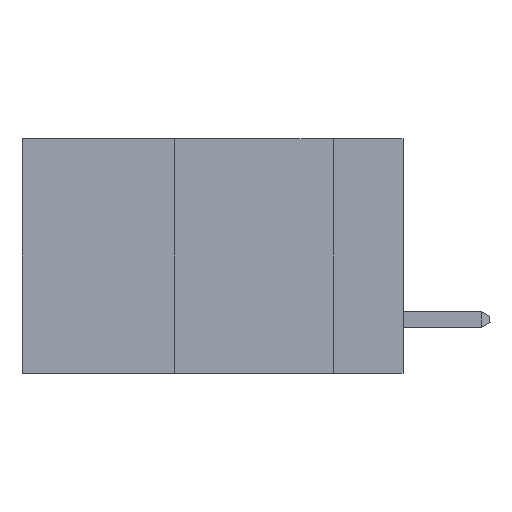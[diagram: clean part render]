
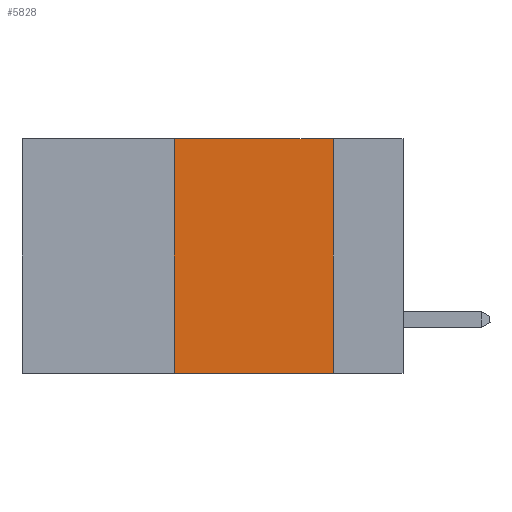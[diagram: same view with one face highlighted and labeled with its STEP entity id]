
A CAD part, left-side view. The second image highlights one B-rep face of the part: STEP entity #5828.
In plain terms, the highlighted planar face has unit normal (-1, 0, 0).
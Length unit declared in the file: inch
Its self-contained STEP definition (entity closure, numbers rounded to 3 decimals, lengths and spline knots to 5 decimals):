
#2307 = CARTESIAN_POINT ( 'NONE',  ( 0., 0.11, 0. ) ) ;
#2425 = CARTESIAN_POINT ( 'NONE',  ( 0., 0.36, 0. ) ) ;
#3149 = CARTESIAN_POINT ( 'NONE',  ( 0., 0.36, -0.37 ) ) ;
#4211 = VERTEX_POINT ( 'NONE', #2425 ) ;
#5221 = VERTEX_POINT ( 'NONE', #33621 ) ;
#5508 = CARTESIAN_POINT ( 'NONE',  ( 0., 0.6, 0. ) ) ;
#5828 = ADVANCED_FACE ( 'NONE', ( #44505 ), #46848, .F. ) ;
#6279 = CARTESIAN_POINT ( 'NONE',  ( 0., 0.11, -0.37 ) ) ;
#8503 = DIRECTION ( 'NONE',  ( 1., 0., 0. ) ) ;
#9434 = ORIENTED_EDGE ( 'NONE', *, *, #49886, .F. ) ;
#10566 = EDGE_CURVE ( 'NONE', #5221, #21000, #13052, .T. ) ;
#12055 = DIRECTION ( 'NONE',  ( 0., -1., 0. ) ) ;
#12700 = VECTOR ( 'NONE', #33296, 39.37008 ) ;
#13052 = LINE ( 'NONE', #2307, #20924 ) ;
#13953 = EDGE_LOOP ( 'NONE', ( #40912, #9434, #32445, #31749 ) ) ;
#14156 = DIRECTION ( 'NONE',  ( 0., 0., -1. ) ) ;
#17093 = EDGE_CURVE ( 'NONE', #43874, #21000, #49268, .T. ) ;
#20924 = VECTOR ( 'NONE', #14156, 39.37008 ) ;
#21000 = VERTEX_POINT ( 'NONE', #6279 ) ;
#21794 = CARTESIAN_POINT ( 'NONE',  ( 0., 0.36, 0. ) ) ;
#24425 = EDGE_CURVE ( 'NONE', #43874, #4211, #36939, .T. ) ;
#27819 = CARTESIAN_POINT ( 'NONE',  ( 0., 0.6, 0. ) ) ;
#29248 = AXIS2_PLACEMENT_3D ( 'NONE', #27819, #8503, #47358 ) ;
#31545 = CARTESIAN_POINT ( 'NONE',  ( 0., 0.6, -0.37 ) ) ;
#31585 = VECTOR ( 'NONE', #12055, 39.37008 ) ;
#31685 = LINE ( 'NONE', #5508, #44494 ) ;
#31749 = ORIENTED_EDGE ( 'NONE', *, *, #17093, .T. ) ;
#32445 = ORIENTED_EDGE ( 'NONE', *, *, #24425, .F. ) ;
#32465 = DIRECTION ( 'NONE',  ( 0., -1., 0. ) ) ;
#33296 = DIRECTION ( 'NONE',  ( 0., 0., 1. ) ) ;
#33621 = CARTESIAN_POINT ( 'NONE',  ( 0., 0.11, 0. ) ) ;
#36939 = LINE ( 'NONE', #21794, #12700 ) ;
#40912 = ORIENTED_EDGE ( 'NONE', *, *, #10566, .F. ) ;
#43874 = VERTEX_POINT ( 'NONE', #3149 ) ;
#44494 = VECTOR ( 'NONE', #32465, 39.37008 ) ;
#44505 = FACE_OUTER_BOUND ( 'NONE', #13953, .T. ) ;
#46848 = PLANE ( 'NONE',  #29248 ) ;
#47358 = DIRECTION ( 'NONE',  ( 0., 0., -1. ) ) ;
#49268 = LINE ( 'NONE', #31545, #31585 ) ;
#49886 = EDGE_CURVE ( 'NONE', #4211, #5221, #31685, .T. ) ;
